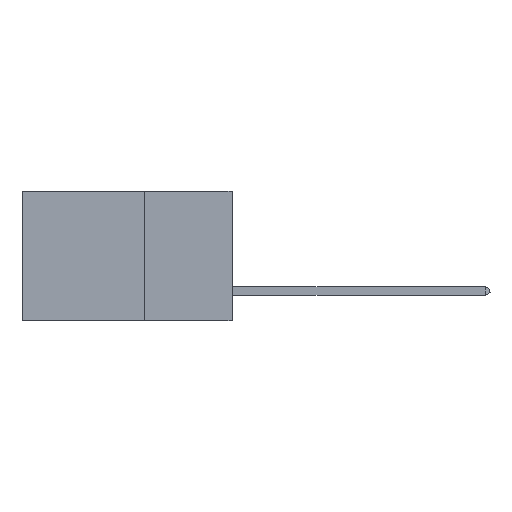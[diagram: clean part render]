
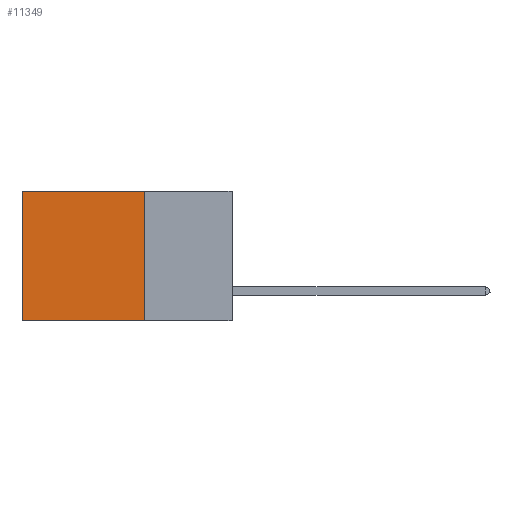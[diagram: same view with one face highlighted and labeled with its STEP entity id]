
A CAD part, left-side view. The second image highlights one B-rep face of the part: STEP entity #11349.
In plain terms, the highlighted planar face has unit normal (-1, 0, 0).
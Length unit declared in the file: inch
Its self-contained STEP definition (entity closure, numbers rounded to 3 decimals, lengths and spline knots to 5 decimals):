
#93 = CARTESIAN_POINT ( 'NONE',  ( 0.2875, 0.25, -0.37 ) ) ;
#398 = DIRECTION ( 'NONE',  ( 1., 0., 0. ) ) ;
#445 = CARTESIAN_POINT ( 'NONE',  ( 0.2875, 0.25, 0. ) ) ;
#717 = FACE_OUTER_BOUND ( 'NONE', #4668, .T. ) ;
#999 = DIRECTION ( 'NONE',  ( 0., 1., 0. ) ) ;
#1978 = CARTESIAN_POINT ( 'NONE',  ( 0.2875, 0.6, -0.37 ) ) ;
#2029 = VERTEX_POINT ( 'NONE', #15083 ) ;
#2119 = DIRECTION ( 'NONE',  ( 0., 0., -1. ) ) ;
#2175 = LINE ( 'NONE', #17506, #12763 ) ;
#3583 = CARTESIAN_POINT ( 'NONE',  ( 0.2875, 0.25, 0. ) ) ;
#3675 = VERTEX_POINT ( 'NONE', #445 ) ;
#3726 = VECTOR ( 'NONE', #2119, 39.37008 ) ;
#4438 = VERTEX_POINT ( 'NONE', #1978 ) ;
#4668 = EDGE_LOOP ( 'NONE', ( #8122, #11631, #6035, #16102 ) ) ;
#6035 = ORIENTED_EDGE ( 'NONE', *, *, #12152, .F. ) ;
#6248 = EDGE_CURVE ( 'NONE', #17302, #4438, #12376, .T. ) ;
#6278 = LINE ( 'NONE', #3583, #3726 ) ;
#7069 = VECTOR ( 'NONE', #13895, 39.37008 ) ;
#7374 = EDGE_CURVE ( 'NONE', #3675, #2029, #2175, .T. ) ;
#7434 = AXIS2_PLACEMENT_3D ( 'NONE', #8620, #398, #10065 ) ;
#8122 = ORIENTED_EDGE ( 'NONE', *, *, #15213, .T. ) ;
#8620 = CARTESIAN_POINT ( 'NONE',  ( 0.2875, 0.25, 0. ) ) ;
#10065 = DIRECTION ( 'NONE',  ( 0., 0., -1. ) ) ;
#11213 = DIRECTION ( 'NONE',  ( 0., 1., 0. ) ) ;
#11349 = ADVANCED_FACE ( 'NONE', ( #717 ), #12736, .F. ) ;
#11631 = ORIENTED_EDGE ( 'NONE', *, *, #6248, .F. ) ;
#12152 = EDGE_CURVE ( 'NONE', #3675, #17302, #6278, .T. ) ;
#12376 = LINE ( 'NONE', #15096, #13434 ) ;
#12551 = CARTESIAN_POINT ( 'NONE',  ( 0.2875, 0.6, 0. ) ) ;
#12736 = PLANE ( 'NONE',  #7434 ) ;
#12763 = VECTOR ( 'NONE', #999, 39.37008 ) ;
#13356 = LINE ( 'NONE', #12551, #7069 ) ;
#13434 = VECTOR ( 'NONE', #11213, 39.37008 ) ;
#13895 = DIRECTION ( 'NONE',  ( 0., 0., -1. ) ) ;
#15083 = CARTESIAN_POINT ( 'NONE',  ( 0.2875, 0.6, 0. ) ) ;
#15096 = CARTESIAN_POINT ( 'NONE',  ( 0.2875, 0.25, -0.37 ) ) ;
#15213 = EDGE_CURVE ( 'NONE', #2029, #4438, #13356, .T. ) ;
#16102 = ORIENTED_EDGE ( 'NONE', *, *, #7374, .T. ) ;
#17302 = VERTEX_POINT ( 'NONE', #93 ) ;
#17506 = CARTESIAN_POINT ( 'NONE',  ( 0.2875, 0.25, 0. ) ) ;
